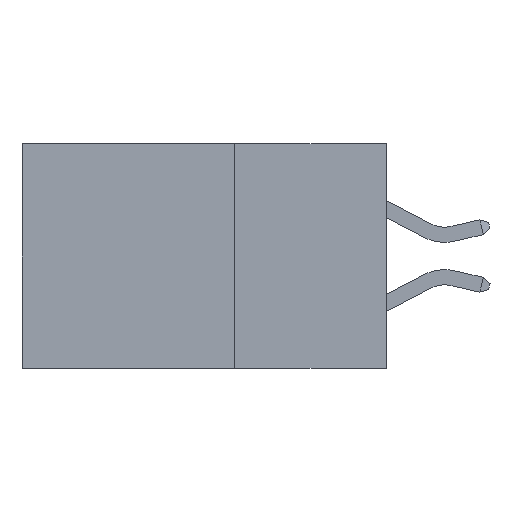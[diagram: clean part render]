
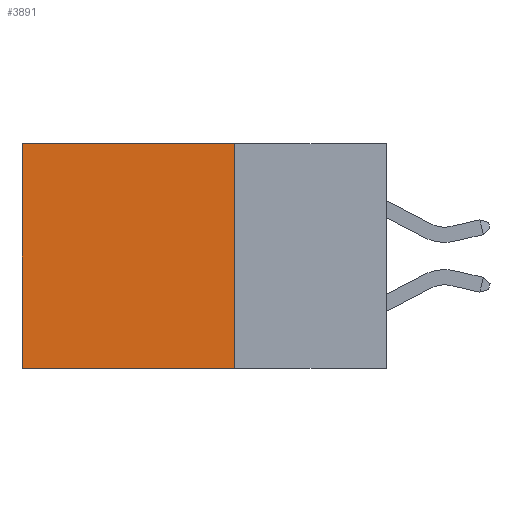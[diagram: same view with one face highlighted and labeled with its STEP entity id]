
A CAD part, left-side view. The second image highlights one B-rep face of the part: STEP entity #3891.
In plain terms, the highlighted planar face has unit normal (-1, 0, 0).
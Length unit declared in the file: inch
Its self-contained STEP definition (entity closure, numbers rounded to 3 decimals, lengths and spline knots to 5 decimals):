
#1641 = LINE ( 'NONE', #14985, #12121 ) ;
#2557 = LINE ( 'NONE', #7505, #6235 ) ;
#3891 = ADVANCED_FACE ( 'NONE', ( #11480 ), #14371, .F. ) ;
#4767 = CARTESIAN_POINT ( 'NONE',  ( 0.2615, 0.25, -0.37 ) ) ;
#4925 = VECTOR ( 'NONE', #14943, 39.37008 ) ;
#5610 = ORIENTED_EDGE ( 'NONE', *, *, #17529, .T. ) ;
#5722 = ORIENTED_EDGE ( 'NONE', *, *, #14545, .F. ) ;
#6128 = DIRECTION ( 'NONE',  ( 0., 1., 0. ) ) ;
#6235 = VECTOR ( 'NONE', #8854, 39.37008 ) ;
#6534 = CARTESIAN_POINT ( 'NONE',  ( 0.2615, 0.25, 0. ) ) ;
#6574 = VERTEX_POINT ( 'NONE', #8913 ) ;
#7353 = EDGE_CURVE ( 'NONE', #11577, #6574, #8480, .T. ) ;
#7505 = CARTESIAN_POINT ( 'NONE',  ( 0.2615, 0.25, -0.37 ) ) ;
#7798 = CARTESIAN_POINT ( 'NONE',  ( 0.2615, 0.6, 0. ) ) ;
#8480 = LINE ( 'NONE', #15355, #4925 ) ;
#8854 = DIRECTION ( 'NONE',  ( 0., 0., -1. ) ) ;
#8913 = CARTESIAN_POINT ( 'NONE',  ( 0.2615, 0.6, -0.37 ) ) ;
#9882 = VECTOR ( 'NONE', #6128, 39.37008 ) ;
#10325 = CARTESIAN_POINT ( 'NONE',  ( 0.2615, 0.25, -0.37 ) ) ;
#11432 = EDGE_CURVE ( 'NONE', #15616, #16126, #2557, .T. ) ;
#11436 = AXIS2_PLACEMENT_3D ( 'NONE', #14391, #14309, #14289 ) ;
#11480 = FACE_OUTER_BOUND ( 'NONE', #14716, .T. ) ;
#11577 = VERTEX_POINT ( 'NONE', #7798 ) ;
#12121 = VECTOR ( 'NONE', #16313, 39.37008 ) ;
#13131 = ORIENTED_EDGE ( 'NONE', *, *, #11432, .F. ) ;
#14289 = DIRECTION ( 'NONE',  ( 0., 0., -1. ) ) ;
#14309 = DIRECTION ( 'NONE',  ( 1., 0., 0. ) ) ;
#14371 = PLANE ( 'NONE',  #11436 ) ;
#14391 = CARTESIAN_POINT ( 'NONE',  ( 0.2615, 0.25, -0.37 ) ) ;
#14545 = EDGE_CURVE ( 'NONE', #16126, #6574, #17447, .T. ) ;
#14716 = EDGE_LOOP ( 'NONE', ( #15642, #5722, #13131, #5610 ) ) ;
#14943 = DIRECTION ( 'NONE',  ( 0., 0., -1. ) ) ;
#14985 = CARTESIAN_POINT ( 'NONE',  ( 0.2615, 0.25, 0. ) ) ;
#15355 = CARTESIAN_POINT ( 'NONE',  ( 0.2615, 0.6, -0.37 ) ) ;
#15616 = VERTEX_POINT ( 'NONE', #6534 ) ;
#15642 = ORIENTED_EDGE ( 'NONE', *, *, #7353, .T. ) ;
#16126 = VERTEX_POINT ( 'NONE', #10325 ) ;
#16313 = DIRECTION ( 'NONE',  ( 0., 1., 0. ) ) ;
#17447 = LINE ( 'NONE', #4767, #9882 ) ;
#17529 = EDGE_CURVE ( 'NONE', #15616, #11577, #1641, .T. ) ;
